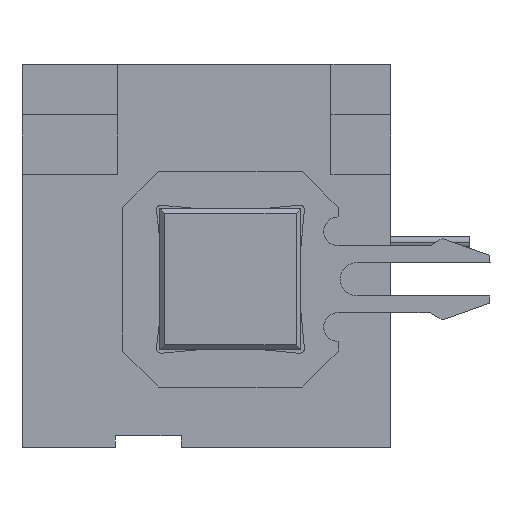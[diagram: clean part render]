
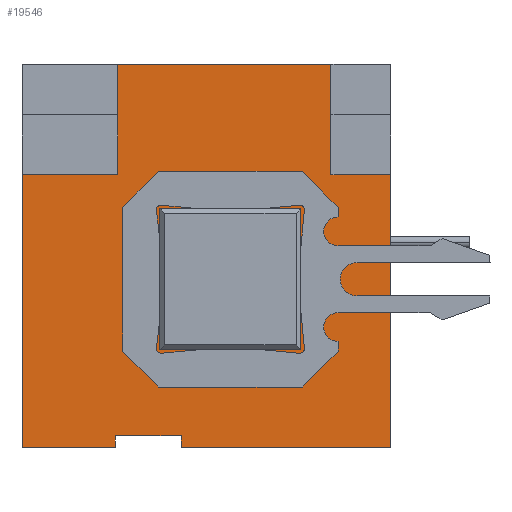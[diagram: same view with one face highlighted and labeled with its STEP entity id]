
A CAD part, left-side view. The second image highlights one B-rep face of the part: STEP entity #19546.
In plain terms, the highlighted planar face has unit normal (-1, 0, 0).
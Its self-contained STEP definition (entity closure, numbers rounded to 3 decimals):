
#103 = EDGE_CURVE ( 'NONE', #2028, #270, #24676, .T. ) ;
#270 = VERTEX_POINT ( 'NONE', #824 ) ;
#634 = CARTESIAN_POINT ( 'NONE',  ( -43.34, 3.755, 9.975 ) ) ;
#824 = CARTESIAN_POINT ( 'NONE',  ( -43.34, 15.4, 11.4 ) ) ;
#881 = ORIENTED_EDGE ( 'NONE', *, *, #103, .F. ) ;
#993 = CARTESIAN_POINT ( 'NONE',  ( -43.34, 9.645, 8. ) ) ;
#1436 = VECTOR ( 'NONE', #24805, 1000. ) ;
#2028 = VERTEX_POINT ( 'NONE', #24539 ) ;
#3030 = ORIENTED_EDGE ( 'NONE', *, *, #35806, .F. ) ;
#4090 = LINE ( 'NONE', #36130, #14873 ) ;
#4247 = PLANE ( 'NONE',  #5345 ) ;
#4266 = CARTESIAN_POINT ( 'NONE',  ( -43.34, 11.5, 0. ) ) ;
#4436 = CARTESIAN_POINT ( 'NONE',  ( -43.34, 2.5, 16. ) ) ;
#4994 = VERTEX_POINT ( 'NONE', #21688 ) ;
#5026 = VERTEX_POINT ( 'NONE', #25619 ) ;
#5233 = EDGE_CURVE ( 'NONE', #5026, #37458, #14880, .T. ) ;
#5345 = AXIS2_PLACEMENT_3D ( 'NONE', #10141, #17344, #13887 ) ;
#5402 = VERTEX_POINT ( 'NONE', #34405 ) ;
#5694 = CARTESIAN_POINT ( 'NONE',  ( -43.34, 11.4, 11.4 ) ) ;
#6515 = DIRECTION ( 'NONE',  ( 0., 0., 1. ) ) ;
#6681 = ORIENTED_EDGE ( 'NONE', *, *, #21541, .F. ) ;
#6755 = EDGE_LOOP ( 'NONE', ( #16425, #6681, #20588, #7333, #17955, #30968, #881, #32483, #7532, #37816, #13733, #24200 ) ) ;
#6795 = VECTOR ( 'NONE', #39220, 1000. ) ;
#7230 = VERTEX_POINT ( 'NONE', #634 ) ;
#7291 = FACE_BOUND ( 'NONE', #38886, .T. ) ;
#7333 = ORIENTED_EDGE ( 'NONE', *, *, #17883, .F. ) ;
#7532 = ORIENTED_EDGE ( 'NONE', *, *, #20923, .T. ) ;
#7601 = DIRECTION ( 'NONE',  ( 0., 0., -1. ) ) ;
#8036 = LINE ( 'NONE', #36391, #13697 ) ;
#8682 = VECTOR ( 'NONE', #6515, 1000. ) ;
#10141 = CARTESIAN_POINT ( 'NONE',  ( -43.34, -0.308, -0.32 ) ) ;
#10165 = CARTESIAN_POINT ( 'NONE',  ( -43.34, 7.7, 16. ) ) ;
#10461 = DIRECTION ( 'NONE',  ( 0., -1., 0. ) ) ;
#10873 = VECTOR ( 'NONE', #39539, 1000. ) ;
#10916 = CARTESIAN_POINT ( 'NONE',  ( -43.34, 8.75, 0.5 ) ) ;
#11216 = LINE ( 'NONE', #37101, #1436 ) ;
#11869 = CARTESIAN_POINT ( 'NONE',  ( -43.34, 11.5, 0.25 ) ) ;
#12959 = VECTOR ( 'NONE', #42106, 1000. ) ;
#13470 = VERTEX_POINT ( 'NONE', #17678 ) ;
#13697 = VECTOR ( 'NONE', #20136, 1000. ) ;
#13733 = ORIENTED_EDGE ( 'NONE', *, *, #31560, .T. ) ;
#13887 = DIRECTION ( 'NONE',  ( 0., 1., 0. ) ) ;
#14379 = DIRECTION ( 'NONE',  ( 0., 0., -1. ) ) ;
#14425 = LINE ( 'NONE', #32783, #26844 ) ;
#14693 = EDGE_CURVE ( 'NONE', #34597, #28333, #8036, .T. ) ;
#14873 = VECTOR ( 'NONE', #22934, 1000. ) ;
#14880 = LINE ( 'NONE', #22838, #21077 ) ;
#15339 = DIRECTION ( 'NONE',  ( 0., 0., 1. ) ) ;
#15647 = CARTESIAN_POINT ( 'NONE',  ( -43.34, 11.5, 0.5 ) ) ;
#16011 = ORIENTED_EDGE ( 'NONE', *, *, #41830, .F. ) ;
#16030 = DIRECTION ( 'NONE',  ( 0., 1., 0. ) ) ;
#16234 = LINE ( 'NONE', #30292, #39029 ) ;
#16425 = ORIENTED_EDGE ( 'NONE', *, *, #19541, .F. ) ;
#17344 = DIRECTION ( 'NONE',  ( 1., 0., 0. ) ) ;
#17377 = ORIENTED_EDGE ( 'NONE', *, *, #28360, .F. ) ;
#17678 = CARTESIAN_POINT ( 'NONE',  ( -43.34, 2.5, 11.4 ) ) ;
#17883 = EDGE_CURVE ( 'NONE', #28333, #29339, #21734, .T. ) ;
#17955 = ORIENTED_EDGE ( 'NONE', *, *, #14693, .F. ) ;
#18709 = CARTESIAN_POINT ( 'NONE',  ( -43.34, 15.4, 8. ) ) ;
#19353 = EDGE_CURVE ( 'NONE', #29339, #13470, #42448, .T. ) ;
#19541 = EDGE_CURVE ( 'NONE', #4994, #5026, #33191, .T. ) ;
#19546 = ADVANCED_FACE ( 'NONE', ( #7291, #23821 ), #4247, .F. ) ;
#19571 = VECTOR ( 'NONE', #16030, 1000. ) ;
#20056 = CARTESIAN_POINT ( 'NONE',  ( -43.34, 3.755, 8. ) ) ;
#20136 = DIRECTION ( 'NONE',  ( 0., 0., 1. ) ) ;
#20588 = ORIENTED_EDGE ( 'NONE', *, *, #19353, .F. ) ;
#20772 = VECTOR ( 'NONE', #7601, 1000. ) ;
#20923 = EDGE_CURVE ( 'NONE', #22496, #34530, #23689, .T. ) ;
#21077 = VECTOR ( 'NONE', #32843, 1000. ) ;
#21509 = VECTOR ( 'NONE', #14379, 1000. ) ;
#21541 = EDGE_CURVE ( 'NONE', #13470, #4994, #4090, .T. ) ;
#21688 = CARTESIAN_POINT ( 'NONE',  ( -43.34, 0., 11.4 ) ) ;
#21734 = LINE ( 'NONE', #10165, #10873 ) ;
#22168 = VECTOR ( 'NONE', #35992, 1000. ) ;
#22496 = VERTEX_POINT ( 'NONE', #4266 ) ;
#22838 = CARTESIAN_POINT ( 'NONE',  ( -43.34, 7.7, 0. ) ) ;
#22934 = DIRECTION ( 'NONE',  ( 0., -1., 0. ) ) ;
#23689 = LINE ( 'NONE', #11869, #24248 ) ;
#23821 = FACE_OUTER_BOUND ( 'NONE', #6755, .T. ) ;
#24200 = ORIENTED_EDGE ( 'NONE', *, *, #5233, .F. ) ;
#24248 = VECTOR ( 'NONE', #15339, 1000. ) ;
#24539 = CARTESIAN_POINT ( 'NONE',  ( -43.34, 15.4, 0. ) ) ;
#24676 = LINE ( 'NONE', #18709, #26766 ) ;
#24805 = DIRECTION ( 'NONE',  ( 0., -1., 0. ) ) ;
#25619 = CARTESIAN_POINT ( 'NONE',  ( -43.34, 0., 0. ) ) ;
#25788 = EDGE_CURVE ( 'NONE', #41374, #34530, #14425, .T. ) ;
#26766 = VECTOR ( 'NONE', #35526, 1000. ) ;
#26844 = VECTOR ( 'NONE', #35701, 1000. ) ;
#27338 = LINE ( 'NONE', #39024, #22168 ) ;
#27573 = CARTESIAN_POINT ( 'NONE',  ( -43.34, 8.75, 0.25 ) ) ;
#27921 = LINE ( 'NONE', #38904, #19571 ) ;
#28333 = VERTEX_POINT ( 'NONE', #36839 ) ;
#28360 = EDGE_CURVE ( 'NONE', #5402, #40507, #41186, .T. ) ;
#29339 = VERTEX_POINT ( 'NONE', #4436 ) ;
#30292 = CARTESIAN_POINT ( 'NONE',  ( -43.34, 7.7, 4.085 ) ) ;
#30968 = ORIENTED_EDGE ( 'NONE', *, *, #42032, .F. ) ;
#31560 = EDGE_CURVE ( 'NONE', #41374, #37458, #34762, .T. ) ;
#32483 = ORIENTED_EDGE ( 'NONE', *, *, #39599, .F. ) ;
#32766 = CARTESIAN_POINT ( 'NONE',  ( -43.34, 3.755, 4.085 ) ) ;
#32783 = CARTESIAN_POINT ( 'NONE',  ( -43.34, 7.7, 0.5 ) ) ;
#32843 = DIRECTION ( 'NONE',  ( 0., 1., 0. ) ) ;
#33191 = LINE ( 'NONE', #35926, #6795 ) ;
#34405 = CARTESIAN_POINT ( 'NONE',  ( -43.34, 9.645, 9.975 ) ) ;
#34530 = VERTEX_POINT ( 'NONE', #15647 ) ;
#34597 = VERTEX_POINT ( 'NONE', #5694 ) ;
#34762 = LINE ( 'NONE', #27573, #20772 ) ;
#35198 = CARTESIAN_POINT ( 'NONE',  ( -43.34, 9.645, 4.085 ) ) ;
#35526 = DIRECTION ( 'NONE',  ( 0., 0., 1. ) ) ;
#35701 = DIRECTION ( 'NONE',  ( 0., 1., 0. ) ) ;
#35806 = EDGE_CURVE ( 'NONE', #40507, #40191, #16234, .T. ) ;
#35926 = CARTESIAN_POINT ( 'NONE',  ( -43.34, 0., 8. ) ) ;
#35992 = DIRECTION ( 'NONE',  ( 0., 1., 0. ) ) ;
#36130 = CARTESIAN_POINT ( 'NONE',  ( -43.34, 7.7, 11.4 ) ) ;
#36391 = CARTESIAN_POINT ( 'NONE',  ( -43.34, 11.4, 8. ) ) ;
#36839 = CARTESIAN_POINT ( 'NONE',  ( -43.34, 11.4, 16. ) ) ;
#37101 = CARTESIAN_POINT ( 'NONE',  ( -43.34, 7.7, 11.4 ) ) ;
#37458 = VERTEX_POINT ( 'NONE', #39812 ) ;
#37620 = LINE ( 'NONE', #20056, #8682 ) ;
#37816 = ORIENTED_EDGE ( 'NONE', *, *, #25788, .F. ) ;
#38886 = EDGE_LOOP ( 'NONE', ( #16011, #3030, #17377, #41295 ) ) ;
#38904 = CARTESIAN_POINT ( 'NONE',  ( -43.34, 7.7, 0. ) ) ;
#39024 = CARTESIAN_POINT ( 'NONE',  ( -43.34, 7.7, 9.975 ) ) ;
#39029 = VECTOR ( 'NONE', #10461, 1000. ) ;
#39220 = DIRECTION ( 'NONE',  ( 0., 0., -1. ) ) ;
#39539 = DIRECTION ( 'NONE',  ( 0., -1., 0. ) ) ;
#39599 = EDGE_CURVE ( 'NONE', #22496, #2028, #27921, .T. ) ;
#39812 = CARTESIAN_POINT ( 'NONE',  ( -43.34, 8.75, 0. ) ) ;
#40191 = VERTEX_POINT ( 'NONE', #32766 ) ;
#40507 = VERTEX_POINT ( 'NONE', #35198 ) ;
#41186 = LINE ( 'NONE', #993, #21509 ) ;
#41212 = EDGE_CURVE ( 'NONE', #7230, #5402, #27338, .T. ) ;
#41295 = ORIENTED_EDGE ( 'NONE', *, *, #41212, .F. ) ;
#41374 = VERTEX_POINT ( 'NONE', #10916 ) ;
#41830 = EDGE_CURVE ( 'NONE', #40191, #7230, #37620, .T. ) ;
#41965 = CARTESIAN_POINT ( 'NONE',  ( -43.34, 2.5, 8. ) ) ;
#42032 = EDGE_CURVE ( 'NONE', #270, #34597, #11216, .T. ) ;
#42106 = DIRECTION ( 'NONE',  ( 0., 0., -1. ) ) ;
#42448 = LINE ( 'NONE', #41965, #12959 ) ;
